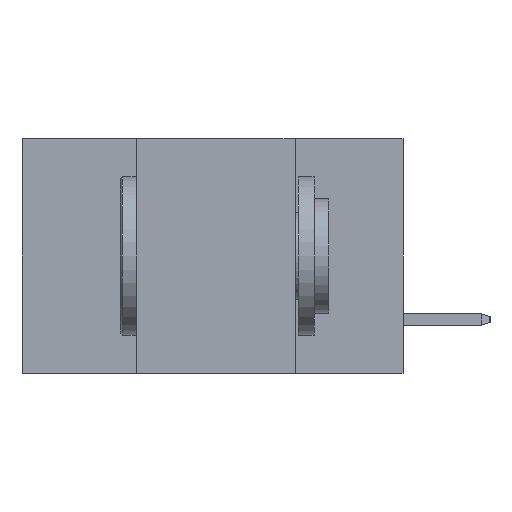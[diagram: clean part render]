
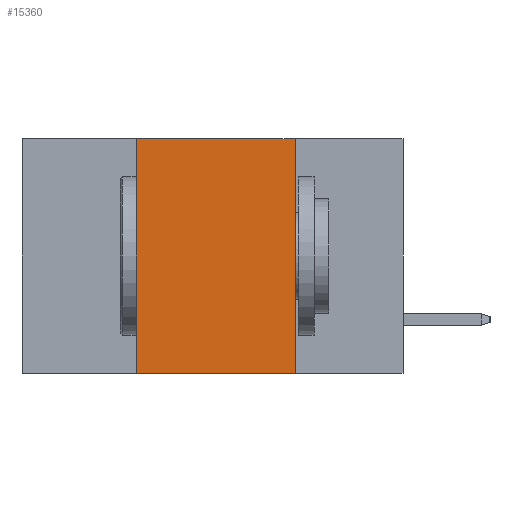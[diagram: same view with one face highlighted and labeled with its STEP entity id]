
A CAD part, left-side view. The second image highlights one B-rep face of the part: STEP entity #15360.
In plain terms, the highlighted planar face has unit normal (-1, 0, 0).
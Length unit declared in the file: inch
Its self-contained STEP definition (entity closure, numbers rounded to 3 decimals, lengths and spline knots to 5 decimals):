
#43 = CARTESIAN_POINT ( 'NONE',  ( 0., 0.42, 0. ) ) ;
#96 = VECTOR ( 'NONE', #8963, 39.37008 ) ;
#910 = VERTEX_POINT ( 'NONE', #3136 ) ;
#1539 = ORIENTED_EDGE ( 'NONE', *, *, #15650, .F. ) ;
#3136 = CARTESIAN_POINT ( 'NONE',  ( 0., 0.42, -0.37 ) ) ;
#3660 = VERTEX_POINT ( 'NONE', #43 ) ;
#3795 = DIRECTION ( 'NONE',  ( 0., -1., 0. ) ) ;
#4059 = EDGE_LOOP ( 'NONE', ( #16503, #5393, #1539, #8330 ) ) ;
#4256 = DIRECTION ( 'NONE',  ( 0., 0., 1. ) ) ;
#5393 = ORIENTED_EDGE ( 'NONE', *, *, #16362, .F. ) ;
#5834 = FACE_OUTER_BOUND ( 'NONE', #4059, .T. ) ;
#7551 = DIRECTION ( 'NONE',  ( 0., -1., 0. ) ) ;
#8049 = VECTOR ( 'NONE', #4256, 39.37008 ) ;
#8330 = ORIENTED_EDGE ( 'NONE', *, *, #11879, .T. ) ;
#8582 = CARTESIAN_POINT ( 'NONE',  ( 0., 0.17, 0. ) ) ;
#8772 = CARTESIAN_POINT ( 'NONE',  ( 0., 0.17, -0.37 ) ) ;
#8878 = CARTESIAN_POINT ( 'NONE',  ( 0., 0.6, -0.37 ) ) ;
#8963 = DIRECTION ( 'NONE',  ( 0., 0., -1. ) ) ;
#9090 = DIRECTION ( 'NONE',  ( 1., 0., 0. ) ) ;
#10377 = CARTESIAN_POINT ( 'NONE',  ( 0., 0.17, 0. ) ) ;
#10645 = VERTEX_POINT ( 'NONE', #8772 ) ;
#10968 = VECTOR ( 'NONE', #7551, 39.37008 ) ;
#11879 = EDGE_CURVE ( 'NONE', #910, #10645, #17695, .T. ) ;
#12429 = VERTEX_POINT ( 'NONE', #8582 ) ;
#13656 = CARTESIAN_POINT ( 'NONE',  ( 0., 0.6, 0. ) ) ;
#13683 = EDGE_CURVE ( 'NONE', #12429, #10645, #15138, .T. ) ;
#15138 = LINE ( 'NONE', #10377, #96 ) ;
#15360 = ADVANCED_FACE ( 'NONE', ( #5834 ), #16987, .F. ) ;
#15650 = EDGE_CURVE ( 'NONE', #910, #3660, #18170, .T. ) ;
#16362 = EDGE_CURVE ( 'NONE', #3660, #12429, #18305, .T. ) ;
#16503 = ORIENTED_EDGE ( 'NONE', *, *, #13683, .F. ) ;
#16589 = CARTESIAN_POINT ( 'NONE',  ( 0., 0.6, 0. ) ) ;
#16987 = PLANE ( 'NONE',  #17077 ) ;
#17077 = AXIS2_PLACEMENT_3D ( 'NONE', #16589, #9090, #18409 ) ;
#17492 = CARTESIAN_POINT ( 'NONE',  ( 0., 0.42, 0. ) ) ;
#17695 = LINE ( 'NONE', #8878, #18584 ) ;
#18170 = LINE ( 'NONE', #17492, #8049 ) ;
#18305 = LINE ( 'NONE', #13656, #10968 ) ;
#18409 = DIRECTION ( 'NONE',  ( 0., 0., -1. ) ) ;
#18584 = VECTOR ( 'NONE', #3795, 39.37008 ) ;
